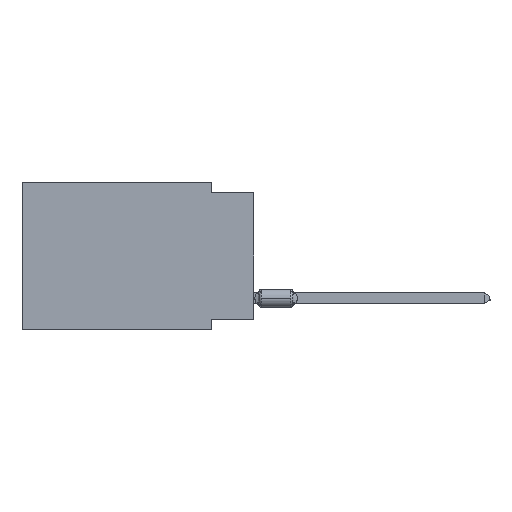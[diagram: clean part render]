
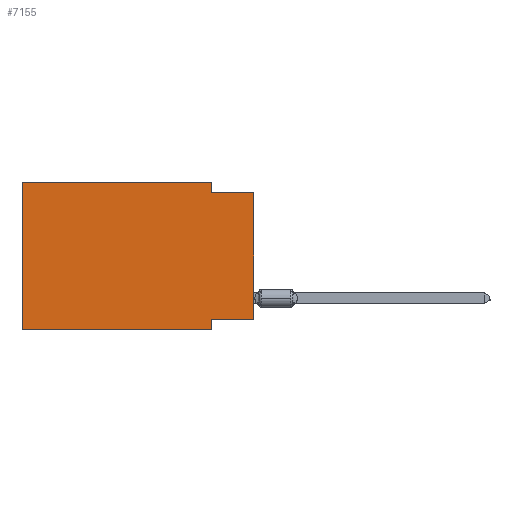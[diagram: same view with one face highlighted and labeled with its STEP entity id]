
A CAD part, left-side view. The second image highlights one B-rep face of the part: STEP entity #7155.
In plain terms, the highlighted planar face has unit normal (-1, 0, 0).
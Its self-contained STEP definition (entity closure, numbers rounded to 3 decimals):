
#368 = EDGE_CURVE ( 'NONE', #44103, #12466, #61239, .T. ) ;
#1035 = LINE ( 'NONE', #67492, #59959 ) ;
#3808 = ORIENTED_EDGE ( 'NONE', *, *, #42217, .T. ) ;
#4083 = VERTEX_POINT ( 'NONE', #47007 ) ;
#4199 = DIRECTION ( 'NONE',  ( 0., 0., 1. ) ) ;
#4775 = CARTESIAN_POINT ( 'NONE',  ( 0., 2.54, 0. ) ) ;
#5361 = CARTESIAN_POINT ( 'NONE',  ( 0., 2.54, -8.89 ) ) ;
#6422 = DIRECTION ( 'NONE',  ( 0., -1., 0. ) ) ;
#6432 = EDGE_CURVE ( 'NONE', #4083, #52720, #1035, .T. ) ;
#6977 = VERTEX_POINT ( 'NONE', #48441 ) ;
#7155 = ADVANCED_FACE ( 'NONE', ( #44820 ), #11604, .F. ) ;
#8993 = DIRECTION ( 'NONE',  ( 0., 0., -1. ) ) ;
#9329 = EDGE_CURVE ( 'NONE', #6977, #30413, #54651, .T. ) ;
#10174 = VECTOR ( 'NONE', #69682, 1000. ) ;
#10309 = CARTESIAN_POINT ( 'NONE',  ( 0., 13.97, -8.89 ) ) ;
#11093 = VECTOR ( 'NONE', #40152, 1000. ) ;
#11604 = PLANE ( 'NONE',  #53186 ) ;
#11915 = VECTOR ( 'NONE', #4199, 1000. ) ;
#11966 = DIRECTION ( 'NONE',  ( 0., 0., -1. ) ) ;
#12466 = VERTEX_POINT ( 'NONE', #27129 ) ;
#14463 = CARTESIAN_POINT ( 'NONE',  ( 0., 0., -8.255 ) ) ;
#14625 = ORIENTED_EDGE ( 'NONE', *, *, #19586, .F. ) ;
#15616 = LINE ( 'NONE', #27035, #11915 ) ;
#17993 = DIRECTION ( 'NONE',  ( 1., 0., 0. ) ) ;
#19586 = EDGE_CURVE ( 'NONE', #30469, #6977, #20349, .T. ) ;
#19689 = LINE ( 'NONE', #24696, #37204 ) ;
#20349 = LINE ( 'NONE', #42147, #10174 ) ;
#21011 = DIRECTION ( 'NONE',  ( 0., -1., 0. ) ) ;
#23727 = EDGE_LOOP ( 'NONE', ( #29762, #64689, #27350, #32653, #51874, #3808, #59560, #14625 ) ) ;
#24696 = CARTESIAN_POINT ( 'NONE',  ( 0., 2.54, 0. ) ) ;
#24856 = VECTOR ( 'NONE', #21011, 1000. ) ;
#27035 = CARTESIAN_POINT ( 'NONE',  ( 0., 0., 0. ) ) ;
#27129 = CARTESIAN_POINT ( 'NONE',  ( 0., 13.97, 0. ) ) ;
#27135 = DIRECTION ( 'NONE',  ( 0., 0., -1. ) ) ;
#27350 = ORIENTED_EDGE ( 'NONE', *, *, #42116, .F. ) ;
#28390 = CARTESIAN_POINT ( 'NONE',  ( 0., 2.54, -8.89 ) ) ;
#29762 = ORIENTED_EDGE ( 'NONE', *, *, #48015, .T. ) ;
#30032 = CARTESIAN_POINT ( 'NONE',  ( 0., 13.97, -8.89 ) ) ;
#30413 = VERTEX_POINT ( 'NONE', #28390 ) ;
#30469 = VERTEX_POINT ( 'NONE', #14463 ) ;
#31379 = CARTESIAN_POINT ( 'NONE',  ( 0., 13.97, 0. ) ) ;
#31742 = EDGE_CURVE ( 'NONE', #12466, #51265, #69645, .T. ) ;
#32653 = ORIENTED_EDGE ( 'NONE', *, *, #31742, .F. ) ;
#35100 = VECTOR ( 'NONE', #27135, 1000. ) ;
#37204 = VECTOR ( 'NONE', #8993, 1000. ) ;
#40152 = DIRECTION ( 'NONE',  ( 0., 0., 1. ) ) ;
#42116 = EDGE_CURVE ( 'NONE', #51265, #4083, #19689, .T. ) ;
#42147 = CARTESIAN_POINT ( 'NONE',  ( 0., 0., -8.255 ) ) ;
#42217 = EDGE_CURVE ( 'NONE', #44103, #30413, #63991, .T. ) ;
#44103 = VERTEX_POINT ( 'NONE', #10309 ) ;
#44820 = FACE_OUTER_BOUND ( 'NONE', #23727, .T. ) ;
#45458 = CARTESIAN_POINT ( 'NONE',  ( 0., 0., -0.635 ) ) ;
#47007 = CARTESIAN_POINT ( 'NONE',  ( 0., 2.54, -0.635 ) ) ;
#48015 = EDGE_CURVE ( 'NONE', #30469, #52720, #15616, .T. ) ;
#48441 = CARTESIAN_POINT ( 'NONE',  ( 0., 2.54, -8.255 ) ) ;
#51265 = VERTEX_POINT ( 'NONE', #4775 ) ;
#51874 = ORIENTED_EDGE ( 'NONE', *, *, #368, .F. ) ;
#52720 = VERTEX_POINT ( 'NONE', #45458 ) ;
#53186 = AXIS2_PLACEMENT_3D ( 'NONE', #66624, #17993, #11966 ) ;
#54651 = LINE ( 'NONE', #5361, #35100 ) ;
#57576 = DIRECTION ( 'NONE',  ( 0., -1., 0. ) ) ;
#59560 = ORIENTED_EDGE ( 'NONE', *, *, #9329, .F. ) ;
#59959 = VECTOR ( 'NONE', #6422, 1000. ) ;
#61239 = LINE ( 'NONE', #67310, #11093 ) ;
#63991 = LINE ( 'NONE', #30032, #70160 ) ;
#64689 = ORIENTED_EDGE ( 'NONE', *, *, #6432, .F. ) ;
#66624 = CARTESIAN_POINT ( 'NONE',  ( 0., 13.97, 0. ) ) ;
#67310 = CARTESIAN_POINT ( 'NONE',  ( 0., 13.97, 0. ) ) ;
#67492 = CARTESIAN_POINT ( 'NONE',  ( 0., 0., -0.635 ) ) ;
#69645 = LINE ( 'NONE', #31379, #24856 ) ;
#69682 = DIRECTION ( 'NONE',  ( 0., 1., 0. ) ) ;
#70160 = VECTOR ( 'NONE', #57576, 1000. ) ;
